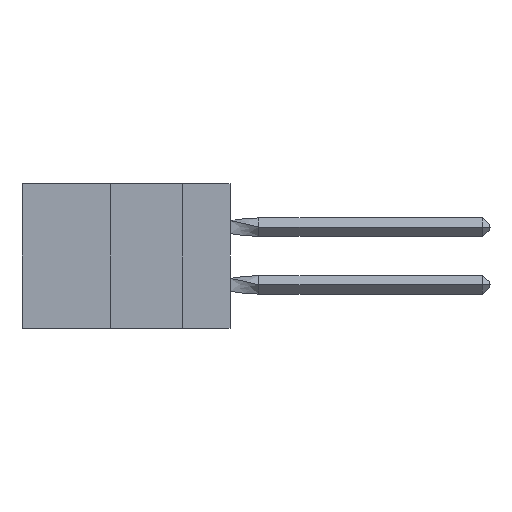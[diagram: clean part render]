
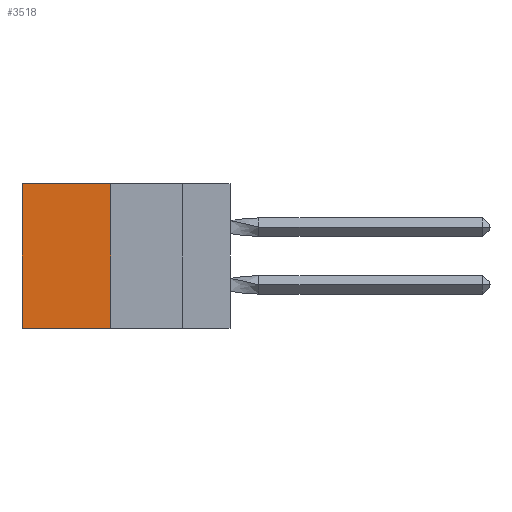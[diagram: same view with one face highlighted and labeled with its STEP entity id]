
A CAD part, left-side view. The second image highlights one B-rep face of the part: STEP entity #3518.
In plain terms, the highlighted planar face has unit normal (-1, 0, 0).
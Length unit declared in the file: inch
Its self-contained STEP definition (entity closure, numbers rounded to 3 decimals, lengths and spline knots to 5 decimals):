
#3518 = ADVANCED_FACE ( 'NONE', ( #27956 ), #20594, .F. ) ;
#3949 = VECTOR ( 'NONE', #27043, 39.37008 ) ;
#4528 = CARTESIAN_POINT ( 'NONE',  ( 0.305, 0.72, 0. ) ) ;
#4760 = DIRECTION ( 'NONE',  ( 1., 0., 0. ) ) ;
#5699 = LINE ( 'NONE', #12269, #28111 ) ;
#6878 = VERTEX_POINT ( 'NONE', #18534 ) ;
#7329 = EDGE_CURVE ( 'NONE', #19527, #26430, #5699, .T. ) ;
#7625 = ORIENTED_EDGE ( 'NONE', *, *, #7329, .T. ) ;
#7654 = CARTESIAN_POINT ( 'NONE',  ( 0.305, 0.413, -0.5 ) ) ;
#10433 = CARTESIAN_POINT ( 'NONE',  ( 0.305, 0.413, -0.5 ) ) ;
#10451 = CARTESIAN_POINT ( 'NONE',  ( 0.305, 0.413, 0. ) ) ;
#11090 = DIRECTION ( 'NONE',  ( 0., 0., -1. ) ) ;
#11784 = LINE ( 'NONE', #7654, #14783 ) ;
#12269 = CARTESIAN_POINT ( 'NONE',  ( 0.305, 0.72, -0.5 ) ) ;
#12723 = CARTESIAN_POINT ( 'NONE',  ( 0.305, 0.413, 0. ) ) ;
#14783 = VECTOR ( 'NONE', #17292, 39.37008 ) ;
#17292 = DIRECTION ( 'NONE',  ( 0., 1., 0. ) ) ;
#18534 = CARTESIAN_POINT ( 'NONE',  ( 0.305, 0.413, -0.5 ) ) ;
#19520 = CARTESIAN_POINT ( 'NONE',  ( 0.305, 0.72, -0.5 ) ) ;
#19527 = VERTEX_POINT ( 'NONE', #4528 ) ;
#20318 = CARTESIAN_POINT ( 'NONE',  ( 0.305, 0.413, -0.5 ) ) ;
#20346 = ORIENTED_EDGE ( 'NONE', *, *, #27984, .F. ) ;
#20594 = PLANE ( 'NONE',  #39018 ) ;
#22583 = ORIENTED_EDGE ( 'NONE', *, *, #37628, .F. ) ;
#26404 = LINE ( 'NONE', #10451, #32877 ) ;
#26430 = VERTEX_POINT ( 'NONE', #19520 ) ;
#26907 = EDGE_CURVE ( 'NONE', #40209, #19527, #26404, .T. ) ;
#27043 = DIRECTION ( 'NONE',  ( 0., 0., -1. ) ) ;
#27956 = FACE_OUTER_BOUND ( 'NONE', #40499, .T. ) ;
#27984 = EDGE_CURVE ( 'NONE', #6878, #26430, #11784, .T. ) ;
#28111 = VECTOR ( 'NONE', #34554, 39.37008 ) ;
#32877 = VECTOR ( 'NONE', #39125, 39.37008 ) ;
#34554 = DIRECTION ( 'NONE',  ( 0., 0., -1. ) ) ;
#36731 = ORIENTED_EDGE ( 'NONE', *, *, #26907, .T. ) ;
#37628 = EDGE_CURVE ( 'NONE', #40209, #6878, #40194, .T. ) ;
#39018 = AXIS2_PLACEMENT_3D ( 'NONE', #10433, #4760, #11090 ) ;
#39125 = DIRECTION ( 'NONE',  ( 0., 1., 0. ) ) ;
#40194 = LINE ( 'NONE', #20318, #3949 ) ;
#40209 = VERTEX_POINT ( 'NONE', #12723 ) ;
#40499 = EDGE_LOOP ( 'NONE', ( #7625, #20346, #22583, #36731 ) ) ;
